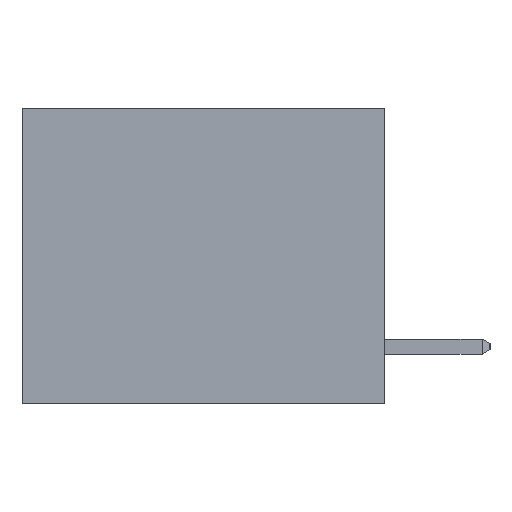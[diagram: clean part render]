
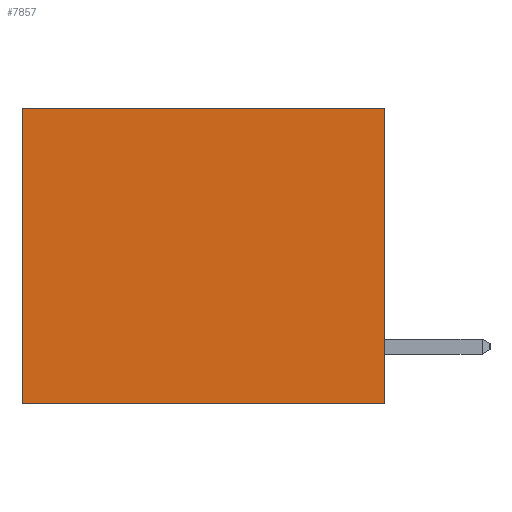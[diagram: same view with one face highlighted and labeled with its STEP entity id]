
A CAD part, left-side view. The second image highlights one B-rep face of the part: STEP entity #7857.
In plain terms, the highlighted planar face has unit normal (-1, 0, 0).
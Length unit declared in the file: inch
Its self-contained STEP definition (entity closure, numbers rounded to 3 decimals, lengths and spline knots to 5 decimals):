
#264 = LINE ( 'NONE', #14394, #3919 ) ;
#825 = CARTESIAN_POINT ( 'NONE',  ( 0.3165, 0., -0.49 ) ) ;
#1478 = EDGE_LOOP ( 'NONE', ( #1834, #21524, #18109, #15286 ) ) ;
#1482 = VECTOR ( 'NONE', #10410, 39.37008 ) ;
#1569 = VECTOR ( 'NONE', #10858, 39.37008 ) ;
#1834 = ORIENTED_EDGE ( 'NONE', *, *, #17817, .T. ) ;
#2066 = CARTESIAN_POINT ( 'NONE',  ( 0.3165, 0., 0. ) ) ;
#3169 = PLANE ( 'NONE',  #28988 ) ;
#3919 = VECTOR ( 'NONE', #9730, 39.37008 ) ;
#4159 = LINE ( 'NONE', #23582, #28285 ) ;
#4391 = EDGE_CURVE ( 'NONE', #16498, #24774, #11464, .T. ) ;
#7545 = VERTEX_POINT ( 'NONE', #16580 ) ;
#7680 = DIRECTION ( 'NONE',  ( 0., 0., -1. ) ) ;
#7857 = ADVANCED_FACE ( 'NONE', ( #25462 ), #3169, .F. ) ;
#9730 = DIRECTION ( 'NONE',  ( 0., 1., 0. ) ) ;
#10410 = DIRECTION ( 'NONE',  ( 0., 1., 0. ) ) ;
#10858 = DIRECTION ( 'NONE',  ( 0., 0., -1. ) ) ;
#11464 = LINE ( 'NONE', #15841, #1569 ) ;
#12272 = DIRECTION ( 'NONE',  ( 0., 0., -1. ) ) ;
#14023 = EDGE_CURVE ( 'NONE', #24774, #7545, #25253, .T. ) ;
#14229 = VERTEX_POINT ( 'NONE', #16012 ) ;
#14394 = CARTESIAN_POINT ( 'NONE',  ( 0.3165, 0., 0. ) ) ;
#15286 = ORIENTED_EDGE ( 'NONE', *, *, #21203, .T. ) ;
#15841 = CARTESIAN_POINT ( 'NONE',  ( 0.3165, 0., -0.49 ) ) ;
#16012 = CARTESIAN_POINT ( 'NONE',  ( 0.3165, 0.6, 0. ) ) ;
#16498 = VERTEX_POINT ( 'NONE', #2066 ) ;
#16580 = CARTESIAN_POINT ( 'NONE',  ( 0.3165, 0.6, -0.49 ) ) ;
#17817 = EDGE_CURVE ( 'NONE', #14229, #7545, #4159, .T. ) ;
#18109 = ORIENTED_EDGE ( 'NONE', *, *, #4391, .F. ) ;
#19506 = DIRECTION ( 'NONE',  ( 1., 0., 0. ) ) ;
#21203 = EDGE_CURVE ( 'NONE', #16498, #14229, #264, .T. ) ;
#21524 = ORIENTED_EDGE ( 'NONE', *, *, #14023, .F. ) ;
#22038 = CARTESIAN_POINT ( 'NONE',  ( 0.3165, 0., -0.49 ) ) ;
#23582 = CARTESIAN_POINT ( 'NONE',  ( 0.3165, 0.6, -0.49 ) ) ;
#24148 = CARTESIAN_POINT ( 'NONE',  ( 0.3165, 0., -0.49 ) ) ;
#24774 = VERTEX_POINT ( 'NONE', #24148 ) ;
#25253 = LINE ( 'NONE', #22038, #1482 ) ;
#25462 = FACE_OUTER_BOUND ( 'NONE', #1478, .T. ) ;
#28285 = VECTOR ( 'NONE', #12272, 39.37008 ) ;
#28988 = AXIS2_PLACEMENT_3D ( 'NONE', #825, #19506, #7680 ) ;
